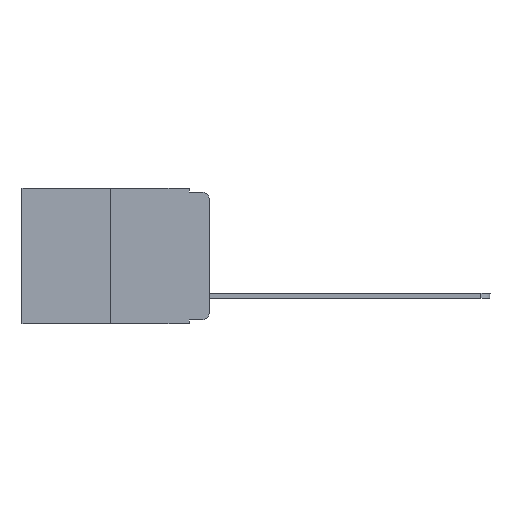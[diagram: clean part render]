
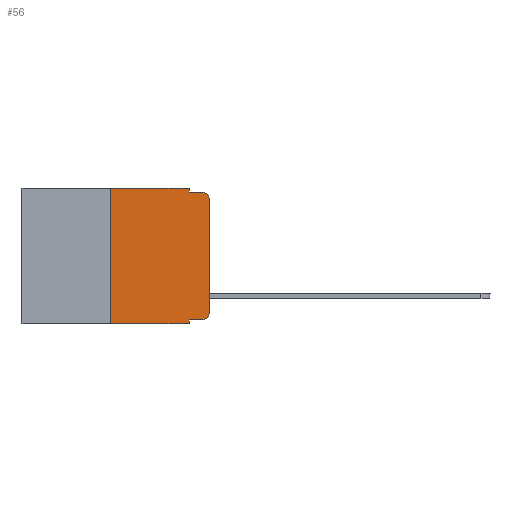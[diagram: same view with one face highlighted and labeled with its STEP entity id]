
A CAD part, left-side view. The second image highlights one B-rep face of the part: STEP entity #56.
In plain terms, the highlighted planar face has unit normal (-1, 0, 0).
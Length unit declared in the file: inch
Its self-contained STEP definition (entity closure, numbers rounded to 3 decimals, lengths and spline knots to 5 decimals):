
#56 = ADVANCED_FACE ( 'NONE', ( #9957 ), #7667, .F. ) ;
#348 = DIRECTION ( 'NONE',  ( 0., -1., 0. ) ) ;
#365 = VECTOR ( 'NONE', #6549, 39.37008 ) ;
#485 = AXIS2_PLACEMENT_3D ( 'NONE', #9996, #1860, #8383 ) ;
#534 = EDGE_CURVE ( 'NONE', #4882, #2527, #10080, .T. ) ;
#662 = EDGE_CURVE ( 'NONE', #8110, #7884, #4805, .T. ) ;
#1018 = EDGE_CURVE ( 'NONE', #7884, #10622, #8034, .T. ) ;
#1019 = CARTESIAN_POINT ( 'NONE',  ( 0., 0.051, -0.333 ) ) ;
#1102 = CARTESIAN_POINT ( 'NONE',  ( 0., 0., -0.313 ) ) ;
#1462 = VERTEX_POINT ( 'NONE', #1019 ) ;
#1524 = EDGE_CURVE ( 'NONE', #6651, #8215, #6498, .T. ) ;
#1688 = EDGE_LOOP ( 'NONE', ( #8604, #6129, #7803, #4026, #3190, #10204, #4768, #4269, #5064, #5378 ) ) ;
#1805 = VECTOR ( 'NONE', #2471, 39.37008 ) ;
#1860 = DIRECTION ( 'NONE',  ( 1., 0., 0. ) ) ;
#1992 = CARTESIAN_POINT ( 'NONE',  ( 0., 0.051, -0.333 ) ) ;
#2026 = DIRECTION ( 'NONE',  ( 0., 0., 1. ) ) ;
#2079 = DIRECTION ( 'NONE',  ( 0., 0., -1. ) ) ;
#2383 = DIRECTION ( 'NONE',  ( 0., -1., 0. ) ) ;
#2471 = DIRECTION ( 'NONE',  ( 0., 0., 1. ) ) ;
#2481 = CARTESIAN_POINT ( 'NONE',  ( 0., 0.02, -0.01 ) ) ;
#2527 = VERTEX_POINT ( 'NONE', #9724 ) ;
#2616 = AXIS2_PLACEMENT_3D ( 'NONE', #5463, #9592, #4669 ) ;
#2885 = EDGE_CURVE ( 'NONE', #4882, #5528, #5809, .T. ) ;
#3190 = ORIENTED_EDGE ( 'NONE', *, *, #6463, .F. ) ;
#3308 = CARTESIAN_POINT ( 'NONE',  ( 0., 0.473, 0. ) ) ;
#3409 = CARTESIAN_POINT ( 'NONE',  ( 0., 0.25, -0.343 ) ) ;
#3432 = VECTOR ( 'NONE', #2026, 39.37008 ) ;
#3602 = CARTESIAN_POINT ( 'NONE',  ( 0., 0.051, -0.01 ) ) ;
#4026 = ORIENTED_EDGE ( 'NONE', *, *, #6585, .F. ) ;
#4269 = ORIENTED_EDGE ( 'NONE', *, *, #8194, .F. ) ;
#4404 = LINE ( 'NONE', #9867, #365 ) ;
#4417 = VERTEX_POINT ( 'NONE', #4698 ) ;
#4669 = DIRECTION ( 'NONE',  ( 0., 0., -1. ) ) ;
#4698 = CARTESIAN_POINT ( 'NONE',  ( 0., 0.051, 0. ) ) ;
#4768 = ORIENTED_EDGE ( 'NONE', *, *, #534, .T. ) ;
#4805 = CIRCLE ( 'NONE', #9717, 0.02 ) ;
#4882 = VERTEX_POINT ( 'NONE', #3409 ) ;
#5064 = ORIENTED_EDGE ( 'NONE', *, *, #9265, .T. ) ;
#5378 = ORIENTED_EDGE ( 'NONE', *, *, #662, .T. ) ;
#5429 = VECTOR ( 'NONE', #348, 39.37008 ) ;
#5463 = CARTESIAN_POINT ( 'NONE',  ( 0., 0.02, -0.03 ) ) ;
#5528 = VERTEX_POINT ( 'NONE', #6259 ) ;
#5717 = VECTOR ( 'NONE', #10217, 39.37008 ) ;
#5809 = LINE ( 'NONE', #6451, #3432 ) ;
#5959 = LINE ( 'NONE', #1992, #5429 ) ;
#6129 = ORIENTED_EDGE ( 'NONE', *, *, #10509, .T. ) ;
#6228 = CARTESIAN_POINT ( 'NONE',  ( 0., 0.051, -0.01 ) ) ;
#6259 = CARTESIAN_POINT ( 'NONE',  ( 0., 0.25, 0. ) ) ;
#6311 = CARTESIAN_POINT ( 'NONE',  ( 0., 0.02, -0.313 ) ) ;
#6342 = CARTESIAN_POINT ( 'NONE',  ( 0., 0.051, 0. ) ) ;
#6451 = CARTESIAN_POINT ( 'NONE',  ( 0., 0.25, 0. ) ) ;
#6463 = EDGE_CURVE ( 'NONE', #5528, #4417, #10372, .T. ) ;
#6498 = LINE ( 'NONE', #3602, #5717 ) ;
#6549 = DIRECTION ( 'NONE',  ( 0., 0., -1. ) ) ;
#6585 = EDGE_CURVE ( 'NONE', #4417, #6651, #8180, .T. ) ;
#6651 = VERTEX_POINT ( 'NONE', #6228 ) ;
#7313 = CARTESIAN_POINT ( 'NONE',  ( 0., 0., -0.03 ) ) ;
#7538 = DIRECTION ( 'NONE',  ( 0., -1., 0. ) ) ;
#7667 = PLANE ( 'NONE',  #485 ) ;
#7803 = ORIENTED_EDGE ( 'NONE', *, *, #1524, .F. ) ;
#7884 = VERTEX_POINT ( 'NONE', #1102 ) ;
#8034 = LINE ( 'NONE', #8998, #1805 ) ;
#8110 = VERTEX_POINT ( 'NONE', #9619 ) ;
#8180 = LINE ( 'NONE', #6342, #9721 ) ;
#8190 = VECTOR ( 'NONE', #7538, 39.37008 ) ;
#8194 = EDGE_CURVE ( 'NONE', #1462, #2527, #4404, .T. ) ;
#8215 = VERTEX_POINT ( 'NONE', #2481 ) ;
#8383 = DIRECTION ( 'NONE',  ( 0., 0., -1. ) ) ;
#8531 = VECTOR ( 'NONE', #2383, 39.37008 ) ;
#8604 = ORIENTED_EDGE ( 'NONE', *, *, #1018, .T. ) ;
#8779 = DIRECTION ( 'NONE',  ( 0., 0., -1. ) ) ;
#8998 = CARTESIAN_POINT ( 'NONE',  ( 0., 0., 0. ) ) ;
#9265 = EDGE_CURVE ( 'NONE', #1462, #8110, #5959, .T. ) ;
#9592 = DIRECTION ( 'NONE',  ( -1., 0., 0. ) ) ;
#9619 = CARTESIAN_POINT ( 'NONE',  ( 0., 0.02, -0.333 ) ) ;
#9676 = CIRCLE ( 'NONE', #2616, 0.02 ) ;
#9717 = AXIS2_PLACEMENT_3D ( 'NONE', #6311, #10519, #8779 ) ;
#9721 = VECTOR ( 'NONE', #2079, 39.37008 ) ;
#9724 = CARTESIAN_POINT ( 'NONE',  ( 0., 0.051, -0.343 ) ) ;
#9867 = CARTESIAN_POINT ( 'NONE',  ( 0., 0.051, 0. ) ) ;
#9957 = FACE_OUTER_BOUND ( 'NONE', #1688, .T. ) ;
#9996 = CARTESIAN_POINT ( 'NONE',  ( 0., 0.473, 0. ) ) ;
#10080 = LINE ( 'NONE', #10533, #8531 ) ;
#10204 = ORIENTED_EDGE ( 'NONE', *, *, #2885, .F. ) ;
#10217 = DIRECTION ( 'NONE',  ( 0., -1., 0. ) ) ;
#10372 = LINE ( 'NONE', #3308, #8190 ) ;
#10509 = EDGE_CURVE ( 'NONE', #10622, #8215, #9676, .T. ) ;
#10519 = DIRECTION ( 'NONE',  ( -1., 0., 0. ) ) ;
#10533 = CARTESIAN_POINT ( 'NONE',  ( 0., 0.473, -0.343 ) ) ;
#10622 = VERTEX_POINT ( 'NONE', #7313 ) ;
